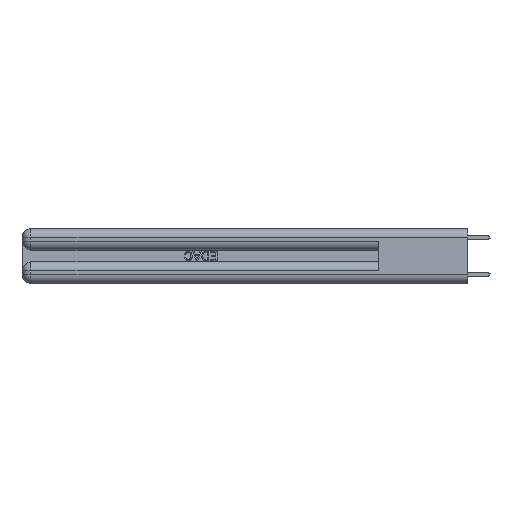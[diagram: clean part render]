
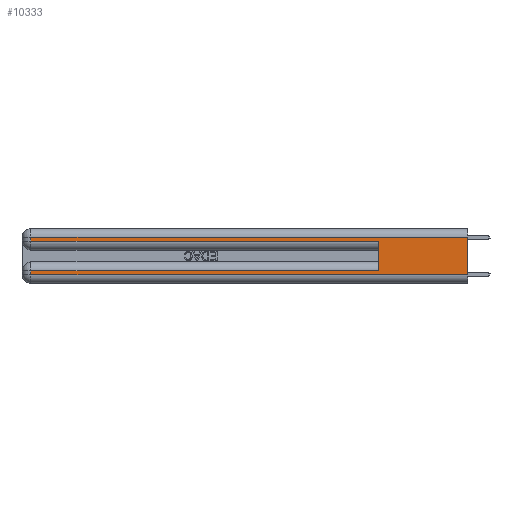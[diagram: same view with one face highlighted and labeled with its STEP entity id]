
A CAD part, left-side view. The second image highlights one B-rep face of the part: STEP entity #10333.
In plain terms, the highlighted planar face has unit normal (-1, 0, 0).
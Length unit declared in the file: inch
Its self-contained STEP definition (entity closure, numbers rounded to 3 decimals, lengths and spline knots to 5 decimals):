
#26 = DIRECTION ( 'NONE',  ( 0., 0., -1. ) ) ;
#426 = VERTEX_POINT ( 'NONE', #5156 ) ;
#958 = DIRECTION ( 'NONE',  ( 1., 0., 0. ) ) ;
#1534 = ORIENTED_EDGE ( 'NONE', *, *, #14493, .T. ) ;
#1559 = CARTESIAN_POINT ( 'NONE',  ( 0., 0., 0.37 ) ) ;
#1822 = CARTESIAN_POINT ( 'NONE',  ( 0., 0., 0.06 ) ) ;
#2729 = FACE_OUTER_BOUND ( 'NONE', #15086, .T. ) ;
#2962 = LINE ( 'NONE', #18854, #33341 ) ;
#2965 = EDGE_CURVE ( 'NONE', #29057, #8104, #11766, .T. ) ;
#3004 = EDGE_CURVE ( 'NONE', #29057, #23390, #31220, .T. ) ;
#3654 = VERTEX_POINT ( 'NONE', #14265 ) ;
#4085 = ORIENTED_EDGE ( 'NONE', *, *, #20877, .T. ) ;
#5156 = CARTESIAN_POINT ( 'NONE',  ( 0., 0.6, 0.085 ) ) ;
#5692 = ORIENTED_EDGE ( 'NONE', *, *, #19074, .T. ) ;
#7259 = VECTOR ( 'NONE', #23333, 39.37008 ) ;
#7454 = VECTOR ( 'NONE', #33981, 39.37008 ) ;
#7814 = LINE ( 'NONE', #15425, #7259 ) ;
#8104 = VERTEX_POINT ( 'NONE', #29553 ) ;
#9142 = AXIS2_PLACEMENT_3D ( 'NONE', #15697, #958, #23623 ) ;
#9724 = CARTESIAN_POINT ( 'NONE',  ( 0., 0., 0.285 ) ) ;
#10152 = CARTESIAN_POINT ( 'NONE',  ( 0., 2.94, 0.085 ) ) ;
#10333 = ADVANCED_FACE ( 'NONE', ( #2729 ), #22193, .F. ) ;
#11766 = LINE ( 'NONE', #1559, #23954 ) ;
#12091 = VECTOR ( 'NONE', #12369, 39.37008 ) ;
#12369 = DIRECTION ( 'NONE',  ( 0., -1., 0. ) ) ;
#12691 = CARTESIAN_POINT ( 'NONE',  ( 0., 0., 0.31 ) ) ;
#12771 = VERTEX_POINT ( 'NONE', #31399 ) ;
#13485 = CARTESIAN_POINT ( 'NONE',  ( 0., 0.6, 0.145 ) ) ;
#13926 = ORIENTED_EDGE ( 'NONE', *, *, #3004, .T. ) ;
#14265 = CARTESIAN_POINT ( 'NONE',  ( 0., 2.94, 0.285 ) ) ;
#14493 = EDGE_CURVE ( 'NONE', #25368, #27359, #2962, .T. ) ;
#14944 = LINE ( 'NONE', #1822, #12091 ) ;
#15031 = CARTESIAN_POINT ( 'NONE',  ( 0., 2.94, 0.37 ) ) ;
#15086 = EDGE_LOOP ( 'NONE', ( #27578, #13926, #4085, #5692, #33835, #25900, #1534, #22133 ) ) ;
#15196 = LINE ( 'NONE', #15031, #18158 ) ;
#15425 = CARTESIAN_POINT ( 'NONE',  ( 0., 0., 0.085 ) ) ;
#15697 = CARTESIAN_POINT ( 'NONE',  ( 0., 0., 0.37 ) ) ;
#18158 = VECTOR ( 'NONE', #25703, 39.37008 ) ;
#18854 = CARTESIAN_POINT ( 'NONE',  ( 0., 2.94, 0.37 ) ) ;
#19074 = EDGE_CURVE ( 'NONE', #3654, #12771, #25407, .T. ) ;
#19238 = EDGE_CURVE ( 'NONE', #426, #12771, #26944, .T. ) ;
#20236 = DIRECTION ( 'NONE',  ( 0., -1., 0. ) ) ;
#20877 = EDGE_CURVE ( 'NONE', #23390, #3654, #15196, .T. ) ;
#20987 = CARTESIAN_POINT ( 'NONE',  ( 0., 2.94, 0.06 ) ) ;
#22133 = ORIENTED_EDGE ( 'NONE', *, *, #33173, .T. ) ;
#22193 = PLANE ( 'NONE',  #9142 ) ;
#23033 = VECTOR ( 'NONE', #20236, 39.37008 ) ;
#23247 = EDGE_CURVE ( 'NONE', #426, #25368, #7814, .T. ) ;
#23333 = DIRECTION ( 'NONE',  ( 0., 1., 0. ) ) ;
#23390 = VERTEX_POINT ( 'NONE', #24001 ) ;
#23623 = DIRECTION ( 'NONE',  ( 0., 0., -1. ) ) ;
#23954 = VECTOR ( 'NONE', #32772, 39.37008 ) ;
#24001 = CARTESIAN_POINT ( 'NONE',  ( 0., 2.94, 0.31 ) ) ;
#24664 = VECTOR ( 'NONE', #31941, 39.37008 ) ;
#25368 = VERTEX_POINT ( 'NONE', #10152 ) ;
#25407 = LINE ( 'NONE', #9724, #23033 ) ;
#25703 = DIRECTION ( 'NONE',  ( 0., 0., -1. ) ) ;
#25900 = ORIENTED_EDGE ( 'NONE', *, *, #23247, .T. ) ;
#26944 = LINE ( 'NONE', #13485, #24664 ) ;
#27359 = VERTEX_POINT ( 'NONE', #20987 ) ;
#27578 = ORIENTED_EDGE ( 'NONE', *, *, #2965, .F. ) ;
#29057 = VERTEX_POINT ( 'NONE', #12691 ) ;
#29553 = CARTESIAN_POINT ( 'NONE',  ( 0., 0., 0.06 ) ) ;
#31220 = LINE ( 'NONE', #33475, #7454 ) ;
#31399 = CARTESIAN_POINT ( 'NONE',  ( 0., 0.6, 0.285 ) ) ;
#31941 = DIRECTION ( 'NONE',  ( 0., 0., 1. ) ) ;
#32772 = DIRECTION ( 'NONE',  ( 0., 0., -1. ) ) ;
#33173 = EDGE_CURVE ( 'NONE', #27359, #8104, #14944, .T. ) ;
#33341 = VECTOR ( 'NONE', #26, 39.37008 ) ;
#33475 = CARTESIAN_POINT ( 'NONE',  ( 0., 0., 0.31 ) ) ;
#33835 = ORIENTED_EDGE ( 'NONE', *, *, #19238, .F. ) ;
#33981 = DIRECTION ( 'NONE',  ( 0., 1., 0. ) ) ;
